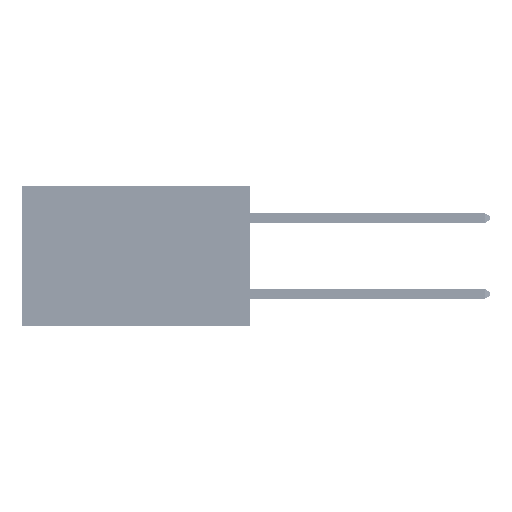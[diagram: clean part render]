
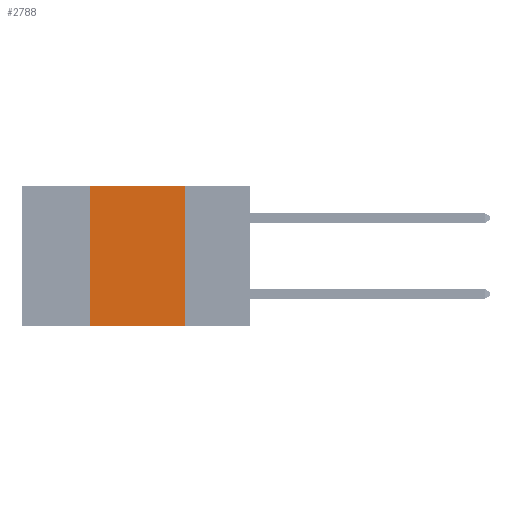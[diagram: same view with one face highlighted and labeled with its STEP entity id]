
A CAD part, left-side view. The second image highlights one B-rep face of the part: STEP entity #2788.
In plain terms, the highlighted planar face has unit normal (-1, 0, 0).
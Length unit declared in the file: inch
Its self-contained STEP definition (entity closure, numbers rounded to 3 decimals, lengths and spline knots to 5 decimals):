
#1648 = CARTESIAN_POINT ( 'NONE',  ( 0., 0.6, 0. ) ) ;
#2788 = ADVANCED_FACE ( 'NONE', ( #13274 ), #42399, .F. ) ;
#4026 = ORIENTED_EDGE ( 'NONE', *, *, #46133, .F. ) ;
#4302 = CARTESIAN_POINT ( 'NONE',  ( 0., 0.17, -0.37 ) ) ;
#4777 = VECTOR ( 'NONE', #39674, 39.37008 ) ;
#6833 = LINE ( 'NONE', #24956, #21429 ) ;
#7632 = EDGE_CURVE ( 'NONE', #9069, #11888, #32632, .T. ) ;
#9069 = VERTEX_POINT ( 'NONE', #27490 ) ;
#9822 = CARTESIAN_POINT ( 'NONE',  ( 0., 0.6, -0.37 ) ) ;
#10336 = DIRECTION ( 'NONE',  ( 0., 0., -1. ) ) ;
#11474 = DIRECTION ( 'NONE',  ( 0., -1., 0. ) ) ;
#11888 = VERTEX_POINT ( 'NONE', #26900 ) ;
#12773 = ORIENTED_EDGE ( 'NONE', *, *, #20840, .F. ) ;
#13123 = CARTESIAN_POINT ( 'NONE',  ( 0., 0.42, -0.37 ) ) ;
#13274 = FACE_OUTER_BOUND ( 'NONE', #18404, .T. ) ;
#15831 = DIRECTION ( 'NONE',  ( 1., 0., 0. ) ) ;
#16626 = AXIS2_PLACEMENT_3D ( 'NONE', #1648, #15831, #23291 ) ;
#17771 = EDGE_CURVE ( 'NONE', #22891, #19805, #34423, .T. ) ;
#18404 = EDGE_LOOP ( 'NONE', ( #12773, #30668, #4026, #31089 ) ) ;
#19805 = VERTEX_POINT ( 'NONE', #4302 ) ;
#20840 = EDGE_CURVE ( 'NONE', #11888, #19805, #6833, .T. ) ;
#21429 = VECTOR ( 'NONE', #10336, 39.37008 ) ;
#22891 = VERTEX_POINT ( 'NONE', #13123 ) ;
#23291 = DIRECTION ( 'NONE',  ( 0., 0., -1. ) ) ;
#24956 = CARTESIAN_POINT ( 'NONE',  ( 0., 0.17, 0. ) ) ;
#25683 = LINE ( 'NONE', #45579, #33822 ) ;
#26900 = CARTESIAN_POINT ( 'NONE',  ( 0., 0.17, 0. ) ) ;
#27490 = CARTESIAN_POINT ( 'NONE',  ( 0., 0.42, 0. ) ) ;
#30316 = VECTOR ( 'NONE', #11474, 39.37008 ) ;
#30513 = DIRECTION ( 'NONE',  ( 0., 0., 1. ) ) ;
#30668 = ORIENTED_EDGE ( 'NONE', *, *, #7632, .F. ) ;
#31089 = ORIENTED_EDGE ( 'NONE', *, *, #17771, .T. ) ;
#32570 = CARTESIAN_POINT ( 'NONE',  ( 0., 0.6, 0. ) ) ;
#32632 = LINE ( 'NONE', #32570, #30316 ) ;
#33822 = VECTOR ( 'NONE', #30513, 39.37008 ) ;
#34423 = LINE ( 'NONE', #9822, #4777 ) ;
#39674 = DIRECTION ( 'NONE',  ( 0., -1., 0. ) ) ;
#42399 = PLANE ( 'NONE',  #16626 ) ;
#45579 = CARTESIAN_POINT ( 'NONE',  ( 0., 0.42, 0. ) ) ;
#46133 = EDGE_CURVE ( 'NONE', #22891, #9069, #25683, .T. ) ;
